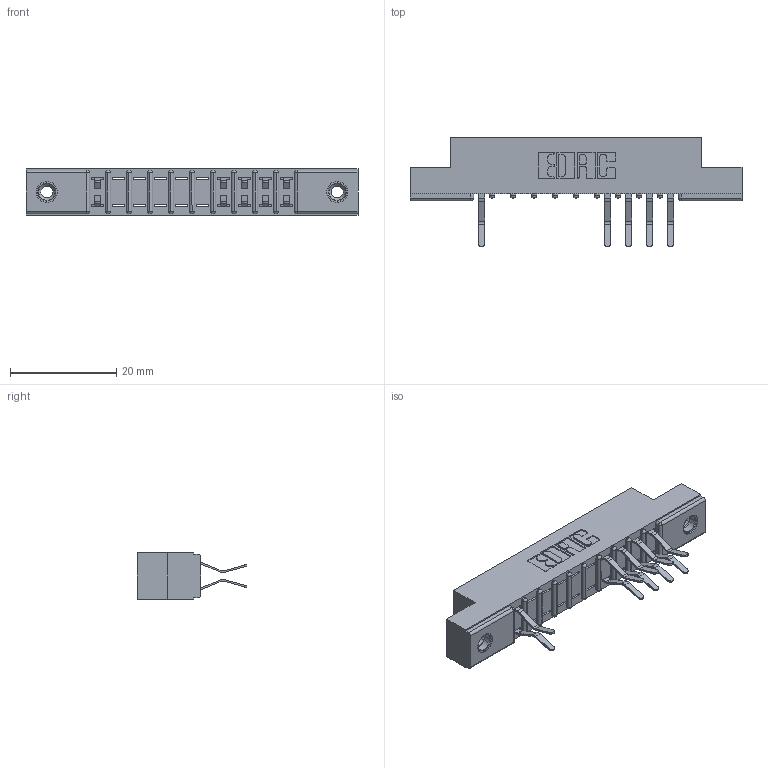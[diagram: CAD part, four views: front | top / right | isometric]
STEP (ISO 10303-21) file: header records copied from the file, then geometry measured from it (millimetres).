
FILE_DESCRIPTION (( 'STEP AP203' ), '1' );
FILE_NAME ('357-020-560-208.STEP', '2018-08-08T09:11:07', ( '' ), ( '' ), 'SwSTEP 2.0', 'SolidWorks 2016', '' );
FILE_SCHEMA (( 'CONFIG_CONTROL_DESIGN' ));
Length unit declared in the file: inch
Products named in the file (4): 307-290-001_560; 345-250-001_345-250-003-102; 357-020-560-208; 307 Part_.156 Dia Mounting Holes
Assembly tree (13 placements, depth 2):
  357-020-560-208
    307 Part_.156 Dia Mounting Holes
    307-290-001_560  x10
    345-250-001_345-250-003-102  x2
Bounding box: 62.64 x 20.73 x 8.71 mm (x, y, z)
Volume: 3974.9 mm3; surface area: 5727.6 mm2
Topology: 13 solids, 13 shells, 789 faces, 2199 edges, 1414 vertices
Faces by surface type: plane 492, cylinder 259, sphere 22, cone 12, torus 4
Entity records: 13807 total; most frequent: CARTESIAN_POINT 2295, ORIENTED_EDGE 2274, DIRECTION 2261, EDGE_CURVE 1137, LINE 857, VECTOR 857, VERTEX_POINT 736, AXIS2_PLACEMENT_3D 702
